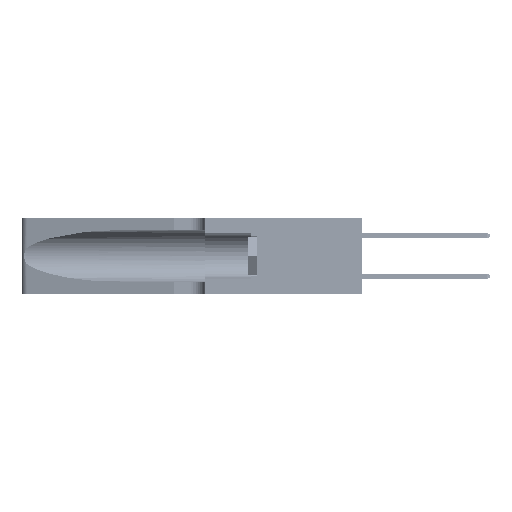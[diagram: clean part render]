
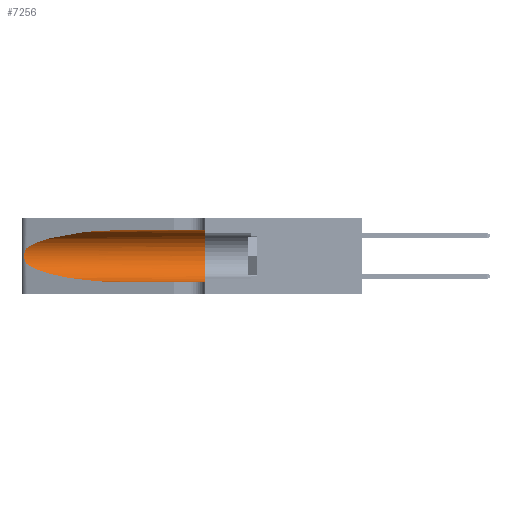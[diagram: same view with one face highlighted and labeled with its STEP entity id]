
A CAD part, left-side view. The second image highlights one B-rep face of the part: STEP entity #7256.
In plain terms, the highlighted cylindrical face has radius 3.308 mm (diameter 6.617 mm), a partial arc.
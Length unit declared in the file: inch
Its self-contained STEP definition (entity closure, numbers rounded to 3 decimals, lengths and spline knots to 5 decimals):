
#78 = VERTEX_POINT ( 'NONE', #35402 ) ;
#1714 = VERTEX_POINT ( 'NONE', #41305 ) ;
#1806 = CARTESIAN_POINT ( 'NONE',  ( 0.2373, 1.15595, 0.08982 ) ) ;
#1983 =( BOUNDED_CURVE ( )  B_SPLINE_CURVE ( 3, ( #33742, #1806, #37734, #13935 ),
 .UNSPECIFIED., .F., .F. ) 
 B_SPLINE_CURVE_WITH_KNOTS ( ( 4, 4 ),
 ( 3.44316, 4.71239 ),
 .UNSPECIFIED. ) 
 CURVE ( )  GEOMETRIC_REPRESENTATION_ITEM ( )  RATIONAL_B_SPLINE_CURVE ( ( 1., 0.87, 0.87, 1. ) ) 
 REPRESENTATION_ITEM ( '' )  );
#3098 = CARTESIAN_POINT ( 'NONE',  ( 0.26018, 1.23835, 0.19895 ) ) ;
#3500 = CARTESIAN_POINT ( 'NONE',  ( 0.1305, 0.72297, 0.31525 ) ) ;
#4218 = CYLINDRICAL_SURFACE ( 'NONE', #8792, 0.13025 ) ;
#5882 = B_SPLINE_CURVE_WITH_KNOTS ( 'NONE', 3,
 ( #30841, #34815, #23053, #50683, #27047, #3098, #31011, #7131, #34990, #11170, #38978, #15202, #42925, #19238 ),
 .UNSPECIFIED., .F., .F.,
 ( 4, 2, 2, 2, 2, 2, 4 ),
 ( 0., 0.00027, 0.00053, 0.00107, 0.0016, 0.00187, 0.00214 ),
 .UNSPECIFIED. ) ;
#7131 = CARTESIAN_POINT ( 'NONE',  ( 0.26075, 1.23896, 0.178 ) ) ;
#7256 = ADVANCED_FACE ( 'NONE', ( #36001 ), #4218, .F. ) ;
#7867 = VERTEX_POINT ( 'NONE', #42599 ) ;
#8792 = AXIS2_PLACEMENT_3D ( 'NONE', #31265, #27297, #19309 ) ;
#10589 = LINE ( 'NONE', #21980, #42276 ) ;
#11170 = CARTESIAN_POINT ( 'NONE',  ( 0.25856, 1.23593, 0.16098 ) ) ;
#11823 = EDGE_CURVE ( 'NONE', #78, #18896, #5882, .T. ) ;
#13446 = CARTESIAN_POINT ( 'NONE',  ( 0.25487, 1.22718, 0.14631 ) ) ;
#13935 = CARTESIAN_POINT ( 'NONE',  ( 0.1305, 0.72297, 0.05475 ) ) ;
#14014 = CARTESIAN_POINT ( 'NONE',  ( 0.1305, 0.72297, 0.31525 ) ) ;
#15202 = CARTESIAN_POINT ( 'NONE',  ( 0.25639, 1.23186, 0.15144 ) ) ;
#15598 = CARTESIAN_POINT ( 'NONE',  ( 0.25487, 1.22718, 0.22369 ) ) ;
#18157 = DIRECTION ( 'NONE',  ( 0., -1., 0. ) ) ;
#18576 = EDGE_CURVE ( 'NONE', #20418, #78, #29859, .T. ) ;
#18896 = VERTEX_POINT ( 'NONE', #13446 ) ;
#19238 = CARTESIAN_POINT ( 'NONE',  ( 0.25487, 1.22718, 0.14631 ) ) ;
#19309 = DIRECTION ( 'NONE',  ( 0., 0., -1. ) ) ;
#20418 = VERTEX_POINT ( 'NONE', #14014 ) ;
#21236 = EDGE_CURVE ( 'NONE', #20418, #7867, #10589, .T. ) ;
#21762 = DIRECTION ( 'NONE',  ( 0., 1., 0. ) ) ;
#21980 = CARTESIAN_POINT ( 'NONE',  ( 0.1305, 1.61858, 0.31525 ) ) ;
#22918 = ORIENTED_EDGE ( 'NONE', *, *, #42438, .F. ) ;
#23053 = CARTESIAN_POINT ( 'NONE',  ( 0.25639, 1.23184, 0.21858 ) ) ;
#24458 = VECTOR ( 'NONE', #46005, 39.37008 ) ;
#26300 = CARTESIAN_POINT ( 'NONE',  ( 0.1305, 1.61858, 0.05475 ) ) ;
#26686 = ORIENTED_EDGE ( 'NONE', *, *, #11823, .T. ) ;
#27047 = CARTESIAN_POINT ( 'NONE',  ( 0.25854, 1.2359, 0.20912 ) ) ;
#27243 = CARTESIAN_POINT ( 'NONE',  ( 0.1305, 0.72297, 0.05475 ) ) ;
#27297 = DIRECTION ( 'NONE',  ( 0., -1., 0. ) ) ;
#27427 = CARTESIAN_POINT ( 'NONE',  ( 0.18966, 0.96281, 0.31525 ) ) ;
#29511 = EDGE_CURVE ( 'NONE', #30635, #1714, #33734, .T. ) ;
#29649 = ORIENTED_EDGE ( 'NONE', *, *, #21236, .F. ) ;
#29859 =( BOUNDED_CURVE ( )  B_SPLINE_CURVE ( 3, ( #3500, #27427, #39369, #15598 ),
 .UNSPECIFIED., .F., .F. ) 
 B_SPLINE_CURVE_WITH_KNOTS ( ( 4, 4 ),
 ( 1.5708, 2.84003 ),
 .UNSPECIFIED. ) 
 CURVE ( )  GEOMETRIC_REPRESENTATION_ITEM ( )  RATIONAL_B_SPLINE_CURVE ( ( 1., 0.87, 0.87, 1. ) ) 
 REPRESENTATION_ITEM ( '' )  );
#30635 = VERTEX_POINT ( 'NONE', #27243 ) ;
#30841 = CARTESIAN_POINT ( 'NONE',  ( 0.25487, 1.22718, 0.22369 ) ) ;
#31011 = CARTESIAN_POINT ( 'NONE',  ( 0.26075, 1.23896, 0.19203 ) ) ;
#31265 = CARTESIAN_POINT ( 'NONE',  ( 0.1305, 1.61858, 0.185 ) ) ;
#33734 = LINE ( 'NONE', #26300, #24458 ) ;
#33742 = CARTESIAN_POINT ( 'NONE',  ( 0.25487, 1.22718, 0.14631 ) ) ;
#34193 = EDGE_LOOP ( 'NONE', ( #42445, #26686, #42255, #51374, #22918, #29649 ) ) ;
#34453 = EDGE_CURVE ( 'NONE', #18896, #30635, #1983, .T. ) ;
#34815 = CARTESIAN_POINT ( 'NONE',  ( 0.25555, 1.22994, 0.2215 ) ) ;
#34990 = CARTESIAN_POINT ( 'NONE',  ( 0.26017, 1.23833, 0.17102 ) ) ;
#35402 = CARTESIAN_POINT ( 'NONE',  ( 0.25487, 1.22718, 0.22369 ) ) ;
#36001 = FACE_OUTER_BOUND ( 'NONE', #34193, .T. ) ;
#37734 = CARTESIAN_POINT ( 'NONE',  ( 0.18966, 0.96281, 0.05475 ) ) ;
#38978 = CARTESIAN_POINT ( 'NONE',  ( 0.25789, 1.23486, 0.15765 ) ) ;
#39369 = CARTESIAN_POINT ( 'NONE',  ( 0.2373, 1.15595, 0.28018 ) ) ;
#41305 = CARTESIAN_POINT ( 'NONE',  ( 0.1305, 0.35, 0.05475 ) ) ;
#41757 = AXIS2_PLACEMENT_3D ( 'NONE', #45449, #21762, #49427 ) ;
#42255 = ORIENTED_EDGE ( 'NONE', *, *, #34453, .T. ) ;
#42276 = VECTOR ( 'NONE', #18157, 39.37008 ) ;
#42438 = EDGE_CURVE ( 'NONE', #7867, #1714, #46493, .T. ) ;
#42445 = ORIENTED_EDGE ( 'NONE', *, *, #18576, .T. ) ;
#42599 = CARTESIAN_POINT ( 'NONE',  ( 0.1305, 0.35, 0.31525 ) ) ;
#42925 = CARTESIAN_POINT ( 'NONE',  ( 0.25555, 1.22993, 0.14849 ) ) ;
#45449 = CARTESIAN_POINT ( 'NONE',  ( 0.1305, 0.35, 0.185 ) ) ;
#46005 = DIRECTION ( 'NONE',  ( 0., -1., 0. ) ) ;
#46493 = CIRCLE ( 'NONE', #41757, 0.13025 ) ;
#49427 = DIRECTION ( 'NONE',  ( 0., 0., 1. ) ) ;
#50683 = CARTESIAN_POINT ( 'NONE',  ( 0.25787, 1.23484, 0.2124 ) ) ;
#51374 = ORIENTED_EDGE ( 'NONE', *, *, #29511, .T. ) ;
